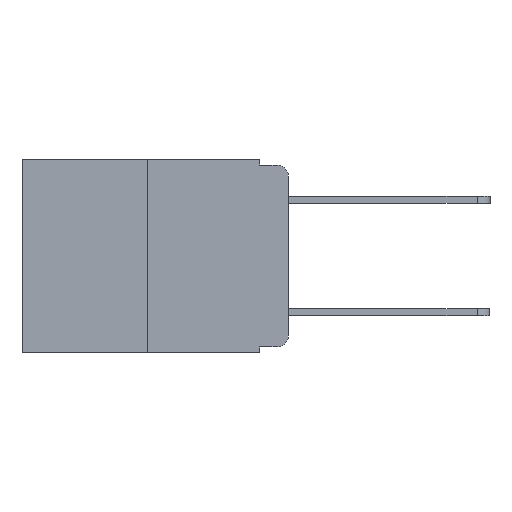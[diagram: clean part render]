
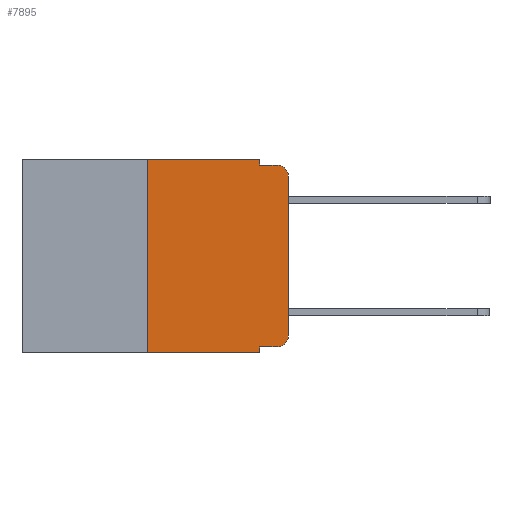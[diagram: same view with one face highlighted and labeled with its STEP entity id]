
A CAD part, left-side view. The second image highlights one B-rep face of the part: STEP entity #7895.
In plain terms, the highlighted planar face has unit normal (-1, 0, 0).
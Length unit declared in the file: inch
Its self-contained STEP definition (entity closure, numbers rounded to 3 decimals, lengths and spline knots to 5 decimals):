
#29 = ORIENTED_EDGE ( 'NONE', *, *, #4450, .F. ) ;
#482 = ORIENTED_EDGE ( 'NONE', *, *, #1738, .T. ) ;
#519 = CARTESIAN_POINT ( 'NONE',  ( 0., 0.051, 0. ) ) ;
#650 = DIRECTION ( 'NONE',  ( 0., 0., -1. ) ) ;
#868 = CIRCLE ( 'NONE', #5856, 0.02 ) ;
#937 = CARTESIAN_POINT ( 'NONE',  ( 0., 0.473, -0.343 ) ) ;
#965 = PLANE ( 'NONE',  #10617 ) ;
#1165 = LINE ( 'NONE', #8005, #2836 ) ;
#1263 = CARTESIAN_POINT ( 'NONE',  ( 0., 0.051, 0. ) ) ;
#1367 = LINE ( 'NONE', #1263, #8781 ) ;
#1394 = VECTOR ( 'NONE', #1589, 39.37008 ) ;
#1488 = EDGE_CURVE ( 'NONE', #5189, #10010, #2699, .T. ) ;
#1589 = DIRECTION ( 'NONE',  ( 0., -1., 0. ) ) ;
#1689 = FACE_OUTER_BOUND ( 'NONE', #9968, .T. ) ;
#1738 = EDGE_CURVE ( 'NONE', #8315, #6596, #1165, .T. ) ;
#1915 = DIRECTION ( 'NONE',  ( 0., -1., 0. ) ) ;
#2151 = EDGE_CURVE ( 'NONE', #5189, #9314, #3959, .T. ) ;
#2390 = CARTESIAN_POINT ( 'NONE',  ( 0., 0.02, -0.333 ) ) ;
#2699 = LINE ( 'NONE', #2846, #7497 ) ;
#2776 = DIRECTION ( 'NONE',  ( 0., -1., 0. ) ) ;
#2789 = EDGE_CURVE ( 'NONE', #9314, #8315, #3800, .T. ) ;
#2801 = ORIENTED_EDGE ( 'NONE', *, *, #6082, .F. ) ;
#2836 = VECTOR ( 'NONE', #8900, 39.37008 ) ;
#2846 = CARTESIAN_POINT ( 'NONE',  ( 0., 0.051, 0. ) ) ;
#2908 = DIRECTION ( 'NONE',  ( 1., 0., 0. ) ) ;
#3244 = ORIENTED_EDGE ( 'NONE', *, *, #4290, .T. ) ;
#3737 = CARTESIAN_POINT ( 'NONE',  ( 0., 0.02, -0.03 ) ) ;
#3800 = CIRCLE ( 'NONE', #11127, 0.02 ) ;
#3959 = LINE ( 'NONE', #4369, #1394 ) ;
#4035 = VECTOR ( 'NONE', #7428, 39.37008 ) ;
#4181 = VECTOR ( 'NONE', #11179, 39.37008 ) ;
#4277 = DIRECTION ( 'NONE',  ( 0., 0., -1. ) ) ;
#4290 = EDGE_CURVE ( 'NONE', #6596, #6761, #868, .T. ) ;
#4369 = CARTESIAN_POINT ( 'NONE',  ( 0., 0.051, -0.333 ) ) ;
#4450 = EDGE_CURVE ( 'NONE', #7557, #5319, #8503, .T. ) ;
#5189 = VERTEX_POINT ( 'NONE', #9252 ) ;
#5319 = VERTEX_POINT ( 'NONE', #519 ) ;
#5591 = ORIENTED_EDGE ( 'NONE', *, *, #10452, .F. ) ;
#5856 = AXIS2_PLACEMENT_3D ( 'NONE', #3737, #6483, #6601 ) ;
#6082 = EDGE_CURVE ( 'NONE', #9299, #6761, #9232, .T. ) ;
#6312 = VERTEX_POINT ( 'NONE', #7758 ) ;
#6401 = LINE ( 'NONE', #9794, #4035 ) ;
#6483 = DIRECTION ( 'NONE',  ( -1., 0., 0. ) ) ;
#6520 = LINE ( 'NONE', #937, #10804 ) ;
#6596 = VERTEX_POINT ( 'NONE', #9081 ) ;
#6601 = DIRECTION ( 'NONE',  ( 0., 0., -1. ) ) ;
#6761 = VERTEX_POINT ( 'NONE', #6848 ) ;
#6848 = CARTESIAN_POINT ( 'NONE',  ( 0., 0.02, -0.01 ) ) ;
#6937 = CARTESIAN_POINT ( 'NONE',  ( 0., 0.051, -0.01 ) ) ;
#7428 = DIRECTION ( 'NONE',  ( 0., 0., 1. ) ) ;
#7497 = VECTOR ( 'NONE', #4277, 39.37008 ) ;
#7557 = VERTEX_POINT ( 'NONE', #10856 ) ;
#7758 = CARTESIAN_POINT ( 'NONE',  ( 0., 0.25, -0.343 ) ) ;
#7895 = ADVANCED_FACE ( 'NONE', ( #1689 ), #965, .F. ) ;
#8005 = CARTESIAN_POINT ( 'NONE',  ( 0., 0., 0. ) ) ;
#8180 = ORIENTED_EDGE ( 'NONE', *, *, #11210, .T. ) ;
#8238 = CARTESIAN_POINT ( 'NONE',  ( 0., 0.473, 0. ) ) ;
#8315 = VERTEX_POINT ( 'NONE', #8706 ) ;
#8435 = DIRECTION ( 'NONE',  ( 0., 0., -1. ) ) ;
#8495 = DIRECTION ( 'NONE',  ( -1., 0., 0. ) ) ;
#8503 = LINE ( 'NONE', #11200, #4181 ) ;
#8667 = ORIENTED_EDGE ( 'NONE', *, *, #1488, .F. ) ;
#8706 = CARTESIAN_POINT ( 'NONE',  ( 0., 0., -0.313 ) ) ;
#8781 = VECTOR ( 'NONE', #650, 39.37008 ) ;
#8850 = ORIENTED_EDGE ( 'NONE', *, *, #8889, .F. ) ;
#8889 = EDGE_CURVE ( 'NONE', #5319, #9299, #1367, .T. ) ;
#8900 = DIRECTION ( 'NONE',  ( 0., 0., 1. ) ) ;
#8986 = CARTESIAN_POINT ( 'NONE',  ( 0., 0.02, -0.313 ) ) ;
#9027 = DIRECTION ( 'NONE',  ( 0., 0., -1. ) ) ;
#9081 = CARTESIAN_POINT ( 'NONE',  ( 0., 0., -0.03 ) ) ;
#9232 = LINE ( 'NONE', #9702, #11261 ) ;
#9252 = CARTESIAN_POINT ( 'NONE',  ( 0., 0.051, -0.333 ) ) ;
#9299 = VERTEX_POINT ( 'NONE', #6937 ) ;
#9314 = VERTEX_POINT ( 'NONE', #2390 ) ;
#9702 = CARTESIAN_POINT ( 'NONE',  ( 0., 0.051, -0.01 ) ) ;
#9794 = CARTESIAN_POINT ( 'NONE',  ( 0., 0.25, 0. ) ) ;
#9968 = EDGE_LOOP ( 'NONE', ( #482, #3244, #2801, #8850, #29, #5591, #8180, #8667, #10622, #10508 ) ) ;
#10010 = VERTEX_POINT ( 'NONE', #10125 ) ;
#10125 = CARTESIAN_POINT ( 'NONE',  ( 0., 0.051, -0.343 ) ) ;
#10452 = EDGE_CURVE ( 'NONE', #6312, #7557, #6401, .T. ) ;
#10508 = ORIENTED_EDGE ( 'NONE', *, *, #2789, .T. ) ;
#10617 = AXIS2_PLACEMENT_3D ( 'NONE', #8238, #2908, #9027 ) ;
#10622 = ORIENTED_EDGE ( 'NONE', *, *, #2151, .T. ) ;
#10804 = VECTOR ( 'NONE', #1915, 39.37008 ) ;
#10856 = CARTESIAN_POINT ( 'NONE',  ( 0., 0.25, 0. ) ) ;
#11127 = AXIS2_PLACEMENT_3D ( 'NONE', #8986, #8495, #8435 ) ;
#11179 = DIRECTION ( 'NONE',  ( 0., -1., 0. ) ) ;
#11200 = CARTESIAN_POINT ( 'NONE',  ( 0., 0.473, 0. ) ) ;
#11210 = EDGE_CURVE ( 'NONE', #6312, #10010, #6520, .T. ) ;
#11261 = VECTOR ( 'NONE', #2776, 39.37008 ) ;
